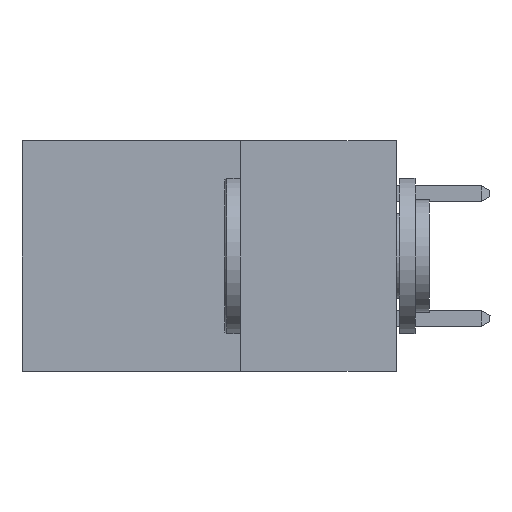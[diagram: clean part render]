
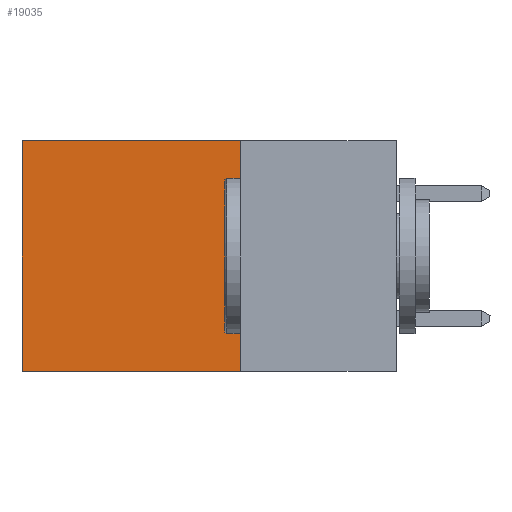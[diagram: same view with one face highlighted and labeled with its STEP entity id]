
A CAD part, left-side view. The second image highlights one B-rep face of the part: STEP entity #19035.
In plain terms, the highlighted planar face has unit normal (-1, 0, 0).
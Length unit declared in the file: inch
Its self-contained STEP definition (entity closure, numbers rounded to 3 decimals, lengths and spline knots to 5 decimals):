
#1497 = AXIS2_PLACEMENT_3D ( 'NONE', #14080, #2375, #16039 ) ;
#1533 = ORIENTED_EDGE ( 'NONE', *, *, #22864, .T. ) ;
#1548 = EDGE_LOOP ( 'NONE', ( #22736, #7145, #5535, #1533 ) ) ;
#2375 = DIRECTION ( 'NONE',  ( 1., 0., 0. ) ) ;
#2933 = CARTESIAN_POINT ( 'NONE',  ( 0.2615, 0.6, -0.37 ) ) ;
#3235 = VECTOR ( 'NONE', #19889, 39.37008 ) ;
#4371 = CARTESIAN_POINT ( 'NONE',  ( 0.2615, 0.25, 0. ) ) ;
#4496 = CARTESIAN_POINT ( 'NONE',  ( 0.2615, 0.25, -0.37 ) ) ;
#5001 = EDGE_CURVE ( 'NONE', #5206, #20506, #11545, .T. ) ;
#5206 = VERTEX_POINT ( 'NONE', #11279 ) ;
#5535 = ORIENTED_EDGE ( 'NONE', *, *, #8895, .F. ) ;
#6479 = DIRECTION ( 'NONE',  ( 0., 0., -1. ) ) ;
#6528 = VERTEX_POINT ( 'NONE', #20740 ) ;
#7145 = ORIENTED_EDGE ( 'NONE', *, *, #5001, .F. ) ;
#8380 = FACE_OUTER_BOUND ( 'NONE', #1548, .T. ) ;
#8439 = LINE ( 'NONE', #4371, #3235 ) ;
#8718 = CARTESIAN_POINT ( 'NONE',  ( 0.2615, 0.25, -0.37 ) ) ;
#8895 = EDGE_CURVE ( 'NONE', #18699, #5206, #17292, .T. ) ;
#10768 = DIRECTION ( 'NONE',  ( 0., 1., 0. ) ) ;
#11279 = CARTESIAN_POINT ( 'NONE',  ( 0.2615, 0.25, -0.37 ) ) ;
#11545 = LINE ( 'NONE', #8718, #21247 ) ;
#13714 = VECTOR ( 'NONE', #22432, 39.37008 ) ;
#14080 = CARTESIAN_POINT ( 'NONE',  ( 0.2615, 0.25, -0.37 ) ) ;
#15704 = EDGE_CURVE ( 'NONE', #6528, #20506, #18896, .T. ) ;
#16039 = DIRECTION ( 'NONE',  ( 0., 0., -1. ) ) ;
#16678 = VECTOR ( 'NONE', #6479, 39.37008 ) ;
#17292 = LINE ( 'NONE', #4496, #16678 ) ;
#18699 = VERTEX_POINT ( 'NONE', #20785 ) ;
#18896 = LINE ( 'NONE', #2933, #13714 ) ;
#19035 = ADVANCED_FACE ( 'NONE', ( #8380 ), #23732, .F. ) ;
#19889 = DIRECTION ( 'NONE',  ( 0., 1., 0. ) ) ;
#20039 = CARTESIAN_POINT ( 'NONE',  ( 0.2615, 0.6, -0.37 ) ) ;
#20506 = VERTEX_POINT ( 'NONE', #20039 ) ;
#20740 = CARTESIAN_POINT ( 'NONE',  ( 0.2615, 0.6, 0. ) ) ;
#20785 = CARTESIAN_POINT ( 'NONE',  ( 0.2615, 0.25, 0. ) ) ;
#21247 = VECTOR ( 'NONE', #10768, 39.37008 ) ;
#22432 = DIRECTION ( 'NONE',  ( 0., 0., -1. ) ) ;
#22736 = ORIENTED_EDGE ( 'NONE', *, *, #15704, .T. ) ;
#22864 = EDGE_CURVE ( 'NONE', #18699, #6528, #8439, .T. ) ;
#23732 = PLANE ( 'NONE',  #1497 ) ;
